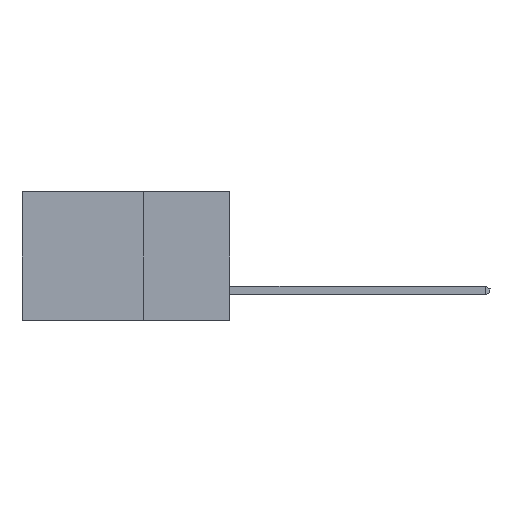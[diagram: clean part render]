
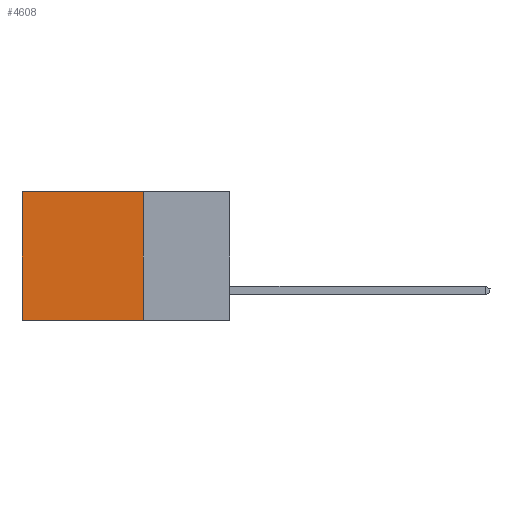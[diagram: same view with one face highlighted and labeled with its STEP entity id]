
A CAD part, left-side view. The second image highlights one B-rep face of the part: STEP entity #4608.
In plain terms, the highlighted planar face has unit normal (-1, 0, 0).
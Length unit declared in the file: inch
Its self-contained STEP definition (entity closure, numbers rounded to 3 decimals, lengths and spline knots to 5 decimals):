
#63 = CARTESIAN_POINT ( 'NONE',  ( 0.2615, 0.25, -0.37 ) ) ;
#180 = CARTESIAN_POINT ( 'NONE',  ( 0.2615, 0.25, 0. ) ) ;
#236 = CARTESIAN_POINT ( 'NONE',  ( 0.2615, 0.6, 0. ) ) ;
#374 = VERTEX_POINT ( 'NONE', #63 ) ;
#620 = LINE ( 'NONE', #7275, #7384 ) ;
#732 = CARTESIAN_POINT ( 'NONE',  ( 0.2615, 0.25, -0.37 ) ) ;
#956 = CARTESIAN_POINT ( 'NONE',  ( 0.2615, 0.6, -0.37 ) ) ;
#1211 = VERTEX_POINT ( 'NONE', #7042 ) ;
#1595 = EDGE_LOOP ( 'NONE', ( #4355, #9659, #5423, #6158 ) ) ;
#1642 = LINE ( 'NONE', #732, #3472 ) ;
#1752 = CARTESIAN_POINT ( 'NONE',  ( 0.2615, 0.25, -0.37 ) ) ;
#2047 = CARTESIAN_POINT ( 'NONE',  ( 0.2615, 0.25, 0. ) ) ;
#3400 = EDGE_CURVE ( 'NONE', #12312, #5591, #11959, .T. ) ;
#3472 = VECTOR ( 'NONE', #7758, 39.37008 ) ;
#4064 = EDGE_CURVE ( 'NONE', #12312, #374, #620, .T. ) ;
#4130 = DIRECTION ( 'NONE',  ( 0., 1., 0. ) ) ;
#4355 = ORIENTED_EDGE ( 'NONE', *, *, #7037, .T. ) ;
#4419 = DIRECTION ( 'NONE',  ( 0., 0., -1. ) ) ;
#4423 = VECTOR ( 'NONE', #4130, 39.37008 ) ;
#4608 = ADVANCED_FACE ( 'NONE', ( #10560 ), #9607, .F. ) ;
#5423 = ORIENTED_EDGE ( 'NONE', *, *, #4064, .F. ) ;
#5591 = VERTEX_POINT ( 'NONE', #236 ) ;
#6158 = ORIENTED_EDGE ( 'NONE', *, *, #3400, .T. ) ;
#6879 = DIRECTION ( 'NONE',  ( 0., 0., -1. ) ) ;
#7037 = EDGE_CURVE ( 'NONE', #5591, #1211, #9772, .T. ) ;
#7042 = CARTESIAN_POINT ( 'NONE',  ( 0.2615, 0.6, -0.37 ) ) ;
#7275 = CARTESIAN_POINT ( 'NONE',  ( 0.2615, 0.25, -0.37 ) ) ;
#7384 = VECTOR ( 'NONE', #4419, 39.37008 ) ;
#7518 = VECTOR ( 'NONE', #6879, 39.37008 ) ;
#7758 = DIRECTION ( 'NONE',  ( 0., 1., 0. ) ) ;
#8251 = AXIS2_PLACEMENT_3D ( 'NONE', #1752, #8651, #8461 ) ;
#8461 = DIRECTION ( 'NONE',  ( 0., 0., -1. ) ) ;
#8651 = DIRECTION ( 'NONE',  ( 1., 0., 0. ) ) ;
#9607 = PLANE ( 'NONE',  #8251 ) ;
#9659 = ORIENTED_EDGE ( 'NONE', *, *, #12562, .F. ) ;
#9772 = LINE ( 'NONE', #956, #7518 ) ;
#10560 = FACE_OUTER_BOUND ( 'NONE', #1595, .T. ) ;
#11959 = LINE ( 'NONE', #180, #4423 ) ;
#12312 = VERTEX_POINT ( 'NONE', #2047 ) ;
#12562 = EDGE_CURVE ( 'NONE', #374, #1211, #1642, .T. ) ;
